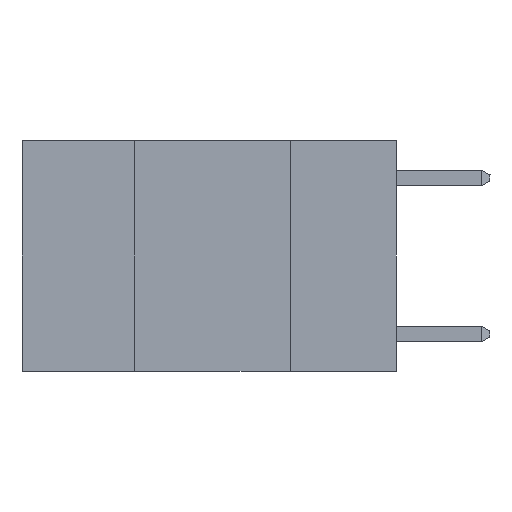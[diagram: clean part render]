
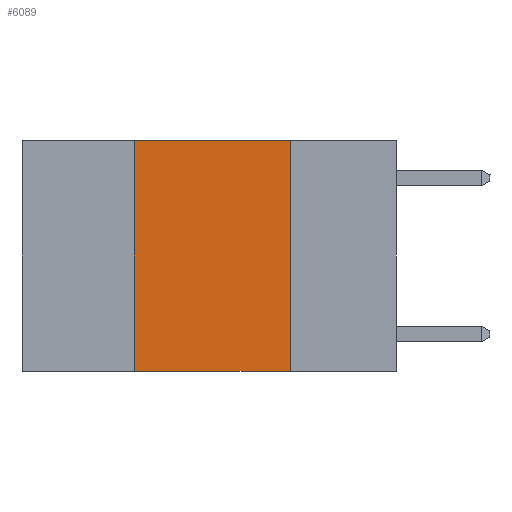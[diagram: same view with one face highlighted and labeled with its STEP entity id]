
A CAD part, left-side view. The second image highlights one B-rep face of the part: STEP entity #6089.
In plain terms, the highlighted planar face has unit normal (-1, 0, 0).
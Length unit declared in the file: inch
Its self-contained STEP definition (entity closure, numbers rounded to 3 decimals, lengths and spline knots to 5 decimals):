
#37 = CARTESIAN_POINT ( 'NONE',  ( 0., 0.17, 0. ) ) ;
#145 = CARTESIAN_POINT ( 'NONE',  ( 0., 0.17, 0. ) ) ;
#361 = VERTEX_POINT ( 'NONE', #5714 ) ;
#479 = ORIENTED_EDGE ( 'NONE', *, *, #1685, .F. ) ;
#734 = DIRECTION ( 'NONE',  ( 0., 0., 1. ) ) ;
#1316 = EDGE_CURVE ( 'NONE', #4802, #2564, #4614, .T. ) ;
#1337 = AXIS2_PLACEMENT_3D ( 'NONE', #4726, #5457, #5292 ) ;
#1685 = EDGE_CURVE ( 'NONE', #3096, #4802, #5129, .T. ) ;
#2092 = PLANE ( 'NONE',  #1337 ) ;
#2095 = ORIENTED_EDGE ( 'NONE', *, *, #1316, .F. ) ;
#2359 = ORIENTED_EDGE ( 'NONE', *, *, #3955, .F. ) ;
#2564 = VERTEX_POINT ( 'NONE', #3954 ) ;
#3096 = VERTEX_POINT ( 'NONE', #6814 ) ;
#3210 = LINE ( 'NONE', #7695, #5456 ) ;
#3226 = DIRECTION ( 'NONE',  ( 0., -1., 0. ) ) ;
#3383 = VECTOR ( 'NONE', #3226, 39.37008 ) ;
#3895 = VECTOR ( 'NONE', #3995, 39.37008 ) ;
#3954 = CARTESIAN_POINT ( 'NONE',  ( 0., 0.17, -0.37 ) ) ;
#3955 = EDGE_CURVE ( 'NONE', #361, #3096, #8049, .T. ) ;
#3995 = DIRECTION ( 'NONE',  ( 0., 0., -1. ) ) ;
#4564 = VECTOR ( 'NONE', #734, 39.37008 ) ;
#4614 = LINE ( 'NONE', #37, #3895 ) ;
#4682 = EDGE_CURVE ( 'NONE', #361, #2564, #3210, .T. ) ;
#4726 = CARTESIAN_POINT ( 'NONE',  ( 0., 0.6, 0. ) ) ;
#4802 = VERTEX_POINT ( 'NONE', #145 ) ;
#4836 = CARTESIAN_POINT ( 'NONE',  ( 0., 0.42, 0. ) ) ;
#5129 = LINE ( 'NONE', #5864, #3383 ) ;
#5292 = DIRECTION ( 'NONE',  ( 0., 0., -1. ) ) ;
#5456 = VECTOR ( 'NONE', #8435, 39.37008 ) ;
#5457 = DIRECTION ( 'NONE',  ( 1., 0., 0. ) ) ;
#5714 = CARTESIAN_POINT ( 'NONE',  ( 0., 0.42, -0.37 ) ) ;
#5864 = CARTESIAN_POINT ( 'NONE',  ( 0., 0.6, 0. ) ) ;
#6089 = ADVANCED_FACE ( 'NONE', ( #7955 ), #2092, .F. ) ;
#6474 = ORIENTED_EDGE ( 'NONE', *, *, #4682, .T. ) ;
#6814 = CARTESIAN_POINT ( 'NONE',  ( 0., 0.42, 0. ) ) ;
#6991 = EDGE_LOOP ( 'NONE', ( #2095, #479, #2359, #6474 ) ) ;
#7695 = CARTESIAN_POINT ( 'NONE',  ( 0., 0.6, -0.37 ) ) ;
#7955 = FACE_OUTER_BOUND ( 'NONE', #6991, .T. ) ;
#8049 = LINE ( 'NONE', #4836, #4564 ) ;
#8435 = DIRECTION ( 'NONE',  ( 0., -1., 0. ) ) ;
